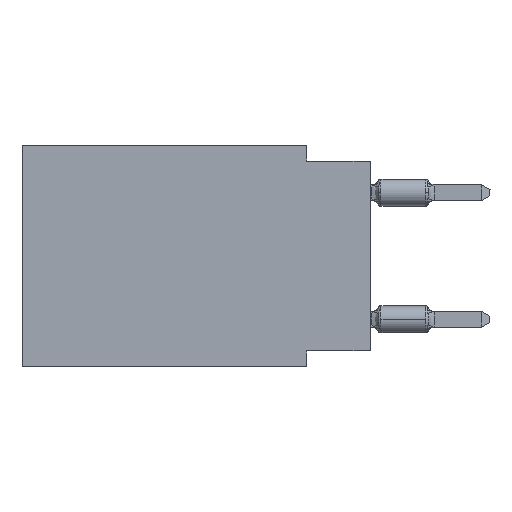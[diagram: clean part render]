
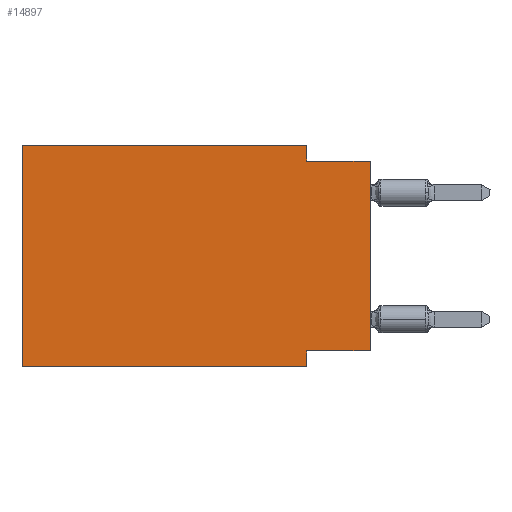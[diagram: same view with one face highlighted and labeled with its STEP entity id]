
A CAD part, left-side view. The second image highlights one B-rep face of the part: STEP entity #14897.
In plain terms, the highlighted planar face has unit normal (-1, 0, 0).
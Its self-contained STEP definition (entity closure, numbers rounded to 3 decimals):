
#1722 = VECTOR ( 'NONE', #29560, 1000. ) ;
#2176 = DIRECTION ( 'NONE',  ( 0., -1., 0. ) ) ;
#2742 = PLANE ( 'NONE',  #38772 ) ;
#2838 = CARTESIAN_POINT ( 'NONE',  ( 0., 2.54, -8.255 ) ) ;
#3009 = VERTEX_POINT ( 'NONE', #49382 ) ;
#3211 = ORIENTED_EDGE ( 'NONE', *, *, #35750, .F. ) ;
#3334 = LINE ( 'NONE', #20194, #4435 ) ;
#3519 = CARTESIAN_POINT ( 'NONE',  ( 0., 2.54, 0. ) ) ;
#4351 = LINE ( 'NONE', #9450, #40379 ) ;
#4435 = VECTOR ( 'NONE', #2176, 1000. ) ;
#7830 = CARTESIAN_POINT ( 'NONE',  ( 0., 0., 0. ) ) ;
#8518 = LINE ( 'NONE', #43146, #11362 ) ;
#8775 = VERTEX_POINT ( 'NONE', #21410 ) ;
#8783 = ORIENTED_EDGE ( 'NONE', *, *, #12432, .F. ) ;
#9066 = DIRECTION ( 'NONE',  ( 0., 0., 1. ) ) ;
#9361 = ORIENTED_EDGE ( 'NONE', *, *, #26379, .F. ) ;
#9450 = CARTESIAN_POINT ( 'NONE',  ( 0., 0., -0.635 ) ) ;
#10456 = DIRECTION ( 'NONE',  ( 0., 0., -1. ) ) ;
#11362 = VECTOR ( 'NONE', #9066, 1000. ) ;
#12131 = EDGE_CURVE ( 'NONE', #49958, #25831, #22142, .T. ) ;
#12219 = CARTESIAN_POINT ( 'NONE',  ( 0., 0., -8.255 ) ) ;
#12432 = EDGE_CURVE ( 'NONE', #48815, #50160, #56447, .T. ) ;
#13651 = CARTESIAN_POINT ( 'NONE',  ( 0., 13.97, 0. ) ) ;
#14897 = ADVANCED_FACE ( 'NONE', ( #50220 ), #2742, .F. ) ;
#15786 = VECTOR ( 'NONE', #25986, 1000. ) ;
#16108 = LINE ( 'NONE', #7830, #43034 ) ;
#17407 = LINE ( 'NONE', #13651, #15786 ) ;
#18163 = ORIENTED_EDGE ( 'NONE', *, *, #20971, .T. ) ;
#19148 = CARTESIAN_POINT ( 'NONE',  ( 0., 2.54, 0. ) ) ;
#20105 = EDGE_LOOP ( 'NONE', ( #18163, #21485, #8783, #3211, #9361, #33658, #33359, #52623 ) ) ;
#20194 = CARTESIAN_POINT ( 'NONE',  ( 0., 13.97, -8.89 ) ) ;
#20971 = EDGE_CURVE ( 'NONE', #40419, #8775, #16108, .T. ) ;
#21410 = CARTESIAN_POINT ( 'NONE',  ( 0., 0., -0.635 ) ) ;
#21485 = ORIENTED_EDGE ( 'NONE', *, *, #40868, .F. ) ;
#21779 = DIRECTION ( 'NONE',  ( 0., -1., 0. ) ) ;
#22142 = LINE ( 'NONE', #39600, #44655 ) ;
#25831 = VERTEX_POINT ( 'NONE', #46348 ) ;
#25986 = DIRECTION ( 'NONE',  ( 0., -1., 0. ) ) ;
#26379 = EDGE_CURVE ( 'NONE', #3009, #34667, #8518, .T. ) ;
#27289 = CARTESIAN_POINT ( 'NONE',  ( 0., 13.97, 0. ) ) ;
#28534 = CARTESIAN_POINT ( 'NONE',  ( 0., 0., -8.255 ) ) ;
#29560 = DIRECTION ( 'NONE',  ( 0., 0., -1. ) ) ;
#33359 = ORIENTED_EDGE ( 'NONE', *, *, #12131, .F. ) ;
#33658 = ORIENTED_EDGE ( 'NONE', *, *, #43378, .T. ) ;
#34667 = VERTEX_POINT ( 'NONE', #27289 ) ;
#35750 = EDGE_CURVE ( 'NONE', #34667, #48815, #17407, .T. ) ;
#36760 = CARTESIAN_POINT ( 'NONE',  ( 0., 13.97, 0. ) ) ;
#36791 = CARTESIAN_POINT ( 'NONE',  ( 0., 2.54, -0.635 ) ) ;
#36809 = DIRECTION ( 'NONE',  ( 0., 1., 0. ) ) ;
#38772 = AXIS2_PLACEMENT_3D ( 'NONE', #36760, #50517, #10456 ) ;
#39600 = CARTESIAN_POINT ( 'NONE',  ( 0., 2.54, -8.89 ) ) ;
#40151 = DIRECTION ( 'NONE',  ( 0., 0., -1. ) ) ;
#40379 = VECTOR ( 'NONE', #21779, 1000. ) ;
#40419 = VERTEX_POINT ( 'NONE', #12219 ) ;
#40868 = EDGE_CURVE ( 'NONE', #50160, #8775, #4351, .T. ) ;
#41402 = LINE ( 'NONE', #28534, #53439 ) ;
#43034 = VECTOR ( 'NONE', #51616, 1000. ) ;
#43146 = CARTESIAN_POINT ( 'NONE',  ( 0., 13.97, 0. ) ) ;
#43378 = EDGE_CURVE ( 'NONE', #3009, #25831, #3334, .T. ) ;
#44655 = VECTOR ( 'NONE', #40151, 1000. ) ;
#46348 = CARTESIAN_POINT ( 'NONE',  ( 0., 2.54, -8.89 ) ) ;
#48815 = VERTEX_POINT ( 'NONE', #19148 ) ;
#49382 = CARTESIAN_POINT ( 'NONE',  ( 0., 13.97, -8.89 ) ) ;
#49958 = VERTEX_POINT ( 'NONE', #2838 ) ;
#50160 = VERTEX_POINT ( 'NONE', #36791 ) ;
#50220 = FACE_OUTER_BOUND ( 'NONE', #20105, .T. ) ;
#50517 = DIRECTION ( 'NONE',  ( 1., 0., 0. ) ) ;
#51616 = DIRECTION ( 'NONE',  ( 0., 0., 1. ) ) ;
#52623 = ORIENTED_EDGE ( 'NONE', *, *, #52802, .F. ) ;
#52802 = EDGE_CURVE ( 'NONE', #40419, #49958, #41402, .T. ) ;
#53439 = VECTOR ( 'NONE', #36809, 1000. ) ;
#56447 = LINE ( 'NONE', #3519, #1722 ) ;
